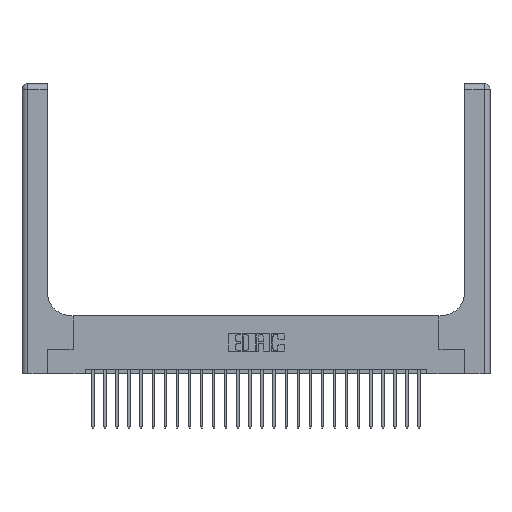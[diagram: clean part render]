
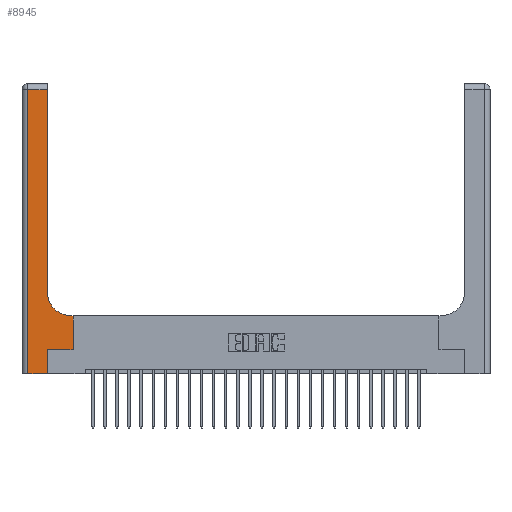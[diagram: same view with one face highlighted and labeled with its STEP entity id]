
A CAD part, top view. The second image highlights one B-rep face of the part: STEP entity #8945.
In plain terms, the highlighted planar face has unit normal (0, 0, 1).
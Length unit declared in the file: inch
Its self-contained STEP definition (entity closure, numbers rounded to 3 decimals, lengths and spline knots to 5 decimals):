
#410 = VERTEX_POINT ( 'NONE', #23779 ) ;
#454 = VECTOR ( 'NONE', #20693, 39.37008 ) ;
#739 = CARTESIAN_POINT ( 'NONE',  ( 0.06, 3., 0.37 ) ) ;
#756 = DIRECTION ( 'NONE',  ( 0., 1., 0. ) ) ;
#950 = CARTESIAN_POINT ( 'NONE',  ( 0.528, 0.6, 0.37 ) ) ;
#1772 = CARTESIAN_POINT ( 'NONE',  ( 0.265, 0., 0.37 ) ) ;
#2024 = DIRECTION ( 'NONE',  ( 0., 0., -1. ) ) ;
#2307 = ORIENTED_EDGE ( 'NONE', *, *, #3227, .T. ) ;
#2324 = VECTOR ( 'NONE', #11875, 39.37008 ) ;
#2404 = CARTESIAN_POINT ( 'NONE',  ( 0.51, 0.85, 0.37 ) ) ;
#2694 = LINE ( 'NONE', #739, #454 ) ;
#3041 = CARTESIAN_POINT ( 'NONE',  ( 0.265, 0., 0.37 ) ) ;
#3227 = EDGE_CURVE ( 'NONE', #13321, #410, #4973, .T. ) ;
#3706 = DIRECTION ( 'NONE',  ( -1., 0., 0. ) ) ;
#3797 = VECTOR ( 'NONE', #11013, 39.37008 ) ;
#4217 = VERTEX_POINT ( 'NONE', #7935 ) ;
#4229 = EDGE_CURVE ( 'NONE', #410, #4217, #7014, .T. ) ;
#4379 = VECTOR ( 'NONE', #15029, 39.37008 ) ;
#4505 = ORIENTED_EDGE ( 'NONE', *, *, #9987, .T. ) ;
#4571 = AXIS2_PLACEMENT_3D ( 'NONE', #19495, #19999, #3706 ) ;
#4709 = CARTESIAN_POINT ( 'NONE',  ( 0.06, 0., 0.37 ) ) ;
#4973 = CIRCLE ( 'NONE', #19956, 0.25 ) ;
#5190 = LINE ( 'NONE', #20839, #7530 ) ;
#5284 = EDGE_CURVE ( 'NONE', #11945, #13321, #11483, .T. ) ;
#5444 = LINE ( 'NONE', #23854, #7995 ) ;
#7014 = LINE ( 'NONE', #13156, #13248 ) ;
#7433 = CARTESIAN_POINT ( 'NONE',  ( 0.265, 0.25, 0.37 ) ) ;
#7530 = VECTOR ( 'NONE', #13038, 39.37008 ) ;
#7794 = ORIENTED_EDGE ( 'NONE', *, *, #19032, .T. ) ;
#7935 = CARTESIAN_POINT ( 'NONE',  ( 0.26, 2.94, 0.37 ) ) ;
#7995 = VECTOR ( 'NONE', #23587, 39.37008 ) ;
#8184 = LINE ( 'NONE', #16163, #23867 ) ;
#8945 = ADVANCED_FACE ( 'NONE', ( #16108 ), #17811, .F. ) ;
#9661 = DIRECTION ( 'NONE',  ( 1., 0., 0. ) ) ;
#9987 = EDGE_CURVE ( 'NONE', #17799, #17725, #5190, .T. ) ;
#10312 = CARTESIAN_POINT ( 'NONE',  ( 0.51, 0.6, 0.37 ) ) ;
#10376 = DIRECTION ( 'NONE',  ( 1., 0., 0. ) ) ;
#10472 = EDGE_CURVE ( 'NONE', #25309, #17799, #23388, .T. ) ;
#11013 = DIRECTION ( 'NONE',  ( 0., 1., 0. ) ) ;
#11428 = EDGE_CURVE ( 'NONE', #17725, #11945, #5444, .T. ) ;
#11483 = LINE ( 'NONE', #23609, #2324 ) ;
#11875 = DIRECTION ( 'NONE',  ( -1., 0., 0. ) ) ;
#11945 = VERTEX_POINT ( 'NONE', #950 ) ;
#12130 = EDGE_CURVE ( 'NONE', #21121, #18972, #2694, .T. ) ;
#13038 = DIRECTION ( 'NONE',  ( 1., 0., 0. ) ) ;
#13123 = ORIENTED_EDGE ( 'NONE', *, *, #4229, .T. ) ;
#13156 = CARTESIAN_POINT ( 'NONE',  ( 0.26, 3., 0.37 ) ) ;
#13248 = VECTOR ( 'NONE', #756, 39.37008 ) ;
#13321 = VERTEX_POINT ( 'NONE', #10312 ) ;
#13716 = EDGE_CURVE ( 'NONE', #18972, #25309, #8184, .T. ) ;
#14593 = ORIENTED_EDGE ( 'NONE', *, *, #12130, .T. ) ;
#15029 = DIRECTION ( 'NONE',  ( -1., 0., 0. ) ) ;
#15349 = ORIENTED_EDGE ( 'NONE', *, *, #10472, .T. ) ;
#15858 = ORIENTED_EDGE ( 'NONE', *, *, #11428, .T. ) ;
#16108 = FACE_OUTER_BOUND ( 'NONE', #16794, .T. ) ;
#16163 = CARTESIAN_POINT ( 'NONE',  ( 0., 0., 0.37 ) ) ;
#16794 = EDGE_LOOP ( 'NONE', ( #13123, #7794, #14593, #21941, #15349, #4505, #15858, #16889, #2307 ) ) ;
#16889 = ORIENTED_EDGE ( 'NONE', *, *, #5284, .T. ) ;
#17266 = CARTESIAN_POINT ( 'NONE',  ( 0., 2.94, 0.37 ) ) ;
#17725 = VERTEX_POINT ( 'NONE', #18946 ) ;
#17799 = VERTEX_POINT ( 'NONE', #7433 ) ;
#17811 = PLANE ( 'NONE',  #4571 ) ;
#18946 = CARTESIAN_POINT ( 'NONE',  ( 0.528, 0.25, 0.37 ) ) ;
#18972 = VERTEX_POINT ( 'NONE', #4709 ) ;
#19032 = EDGE_CURVE ( 'NONE', #4217, #21121, #23238, .T. ) ;
#19495 = CARTESIAN_POINT ( 'NONE',  ( 0., 3., 0.37 ) ) ;
#19956 = AXIS2_PLACEMENT_3D ( 'NONE', #2404, #2024, #10376 ) ;
#19999 = DIRECTION ( 'NONE',  ( 0., 0., -1. ) ) ;
#20693 = DIRECTION ( 'NONE',  ( 0., -1., 0. ) ) ;
#20839 = CARTESIAN_POINT ( 'NONE',  ( 0.265, 0.25, 0.37 ) ) ;
#21121 = VERTEX_POINT ( 'NONE', #21685 ) ;
#21685 = CARTESIAN_POINT ( 'NONE',  ( 0.06, 2.94, 0.37 ) ) ;
#21941 = ORIENTED_EDGE ( 'NONE', *, *, #13716, .T. ) ;
#23238 = LINE ( 'NONE', #17266, #4379 ) ;
#23388 = LINE ( 'NONE', #3041, #3797 ) ;
#23587 = DIRECTION ( 'NONE',  ( 0., 1., 0. ) ) ;
#23609 = CARTESIAN_POINT ( 'NONE',  ( 0.26, 0.6, 0.37 ) ) ;
#23779 = CARTESIAN_POINT ( 'NONE',  ( 0.26, 0.85, 0.37 ) ) ;
#23854 = CARTESIAN_POINT ( 'NONE',  ( 0.528, 0.25, 0.37 ) ) ;
#23867 = VECTOR ( 'NONE', #9661, 39.37008 ) ;
#25309 = VERTEX_POINT ( 'NONE', #1772 ) ;
